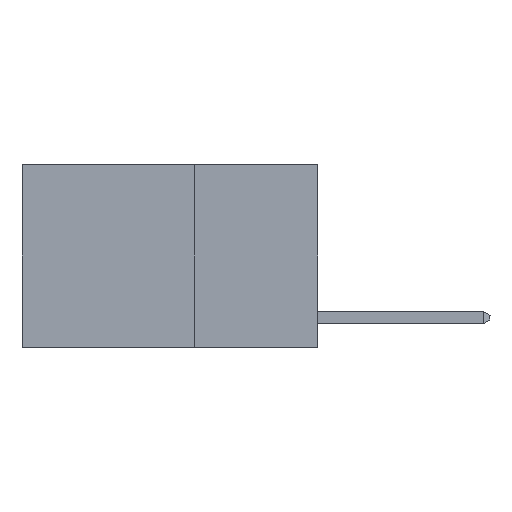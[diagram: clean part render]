
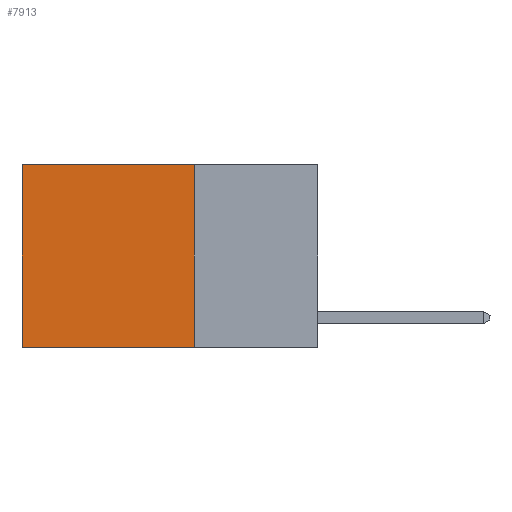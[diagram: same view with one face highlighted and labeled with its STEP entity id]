
A CAD part, left-side view. The second image highlights one B-rep face of the part: STEP entity #7913.
In plain terms, the highlighted planar face has unit normal (-1, 0, 0).
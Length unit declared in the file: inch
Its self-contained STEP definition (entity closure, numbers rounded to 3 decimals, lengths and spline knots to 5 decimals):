
#851 = ORIENTED_EDGE ( 'NONE', *, *, #12708, .T. ) ;
#1005 = CARTESIAN_POINT ( 'NONE',  ( 0.2625, 0.25, -0.37 ) ) ;
#1286 = CARTESIAN_POINT ( 'NONE',  ( 0.2625, 0.25, -0.37 ) ) ;
#2167 = VECTOR ( 'NONE', #9205, 39.37008 ) ;
#2909 = VERTEX_POINT ( 'NONE', #11297 ) ;
#4372 = CARTESIAN_POINT ( 'NONE',  ( 0.2625, 0.6, 0. ) ) ;
#4394 = DIRECTION ( 'NONE',  ( 1., 0., 0. ) ) ;
#4705 = DIRECTION ( 'NONE',  ( 0., 1., 0. ) ) ;
#5455 = DIRECTION ( 'NONE',  ( 0., 0., -1. ) ) ;
#5670 = VECTOR ( 'NONE', #11930, 39.37008 ) ;
#6147 = AXIS2_PLACEMENT_3D ( 'NONE', #6603, #4394, #5455 ) ;
#6603 = CARTESIAN_POINT ( 'NONE',  ( 0.2625, 0.25, 0. ) ) ;
#6653 = EDGE_LOOP ( 'NONE', ( #851, #9534, #7781, #8120 ) ) ;
#6684 = VERTEX_POINT ( 'NONE', #1005 ) ;
#6795 = EDGE_CURVE ( 'NONE', #8015, #2909, #12726, .T. ) ;
#6976 = VERTEX_POINT ( 'NONE', #7713 ) ;
#7713 = CARTESIAN_POINT ( 'NONE',  ( 0.2625, 0.6, -0.37 ) ) ;
#7781 = ORIENTED_EDGE ( 'NONE', *, *, #9267, .F. ) ;
#7913 = ADVANCED_FACE ( 'NONE', ( #10133 ), #10506, .F. ) ;
#7985 = VECTOR ( 'NONE', #4705, 39.37008 ) ;
#7996 = CARTESIAN_POINT ( 'NONE',  ( 0.2625, 0.25, 0. ) ) ;
#8015 = VERTEX_POINT ( 'NONE', #11838 ) ;
#8088 = CARTESIAN_POINT ( 'NONE',  ( 0.2625, 0.25, 0. ) ) ;
#8120 = ORIENTED_EDGE ( 'NONE', *, *, #6795, .T. ) ;
#8486 = VECTOR ( 'NONE', #11857, 39.37008 ) ;
#8582 = EDGE_CURVE ( 'NONE', #6684, #6976, #10270, .T. ) ;
#9094 = LINE ( 'NONE', #4372, #8486 ) ;
#9205 = DIRECTION ( 'NONE',  ( 0., 1., 0. ) ) ;
#9267 = EDGE_CURVE ( 'NONE', #8015, #6684, #11201, .T. ) ;
#9534 = ORIENTED_EDGE ( 'NONE', *, *, #8582, .F. ) ;
#10133 = FACE_OUTER_BOUND ( 'NONE', #6653, .T. ) ;
#10270 = LINE ( 'NONE', #1286, #2167 ) ;
#10506 = PLANE ( 'NONE',  #6147 ) ;
#11201 = LINE ( 'NONE', #7996, #5670 ) ;
#11297 = CARTESIAN_POINT ( 'NONE',  ( 0.2625, 0.6, 0. ) ) ;
#11838 = CARTESIAN_POINT ( 'NONE',  ( 0.2625, 0.25, 0. ) ) ;
#11857 = DIRECTION ( 'NONE',  ( 0., 0., -1. ) ) ;
#11930 = DIRECTION ( 'NONE',  ( 0., 0., -1. ) ) ;
#12708 = EDGE_CURVE ( 'NONE', #2909, #6976, #9094, .T. ) ;
#12726 = LINE ( 'NONE', #8088, #7985 ) ;
